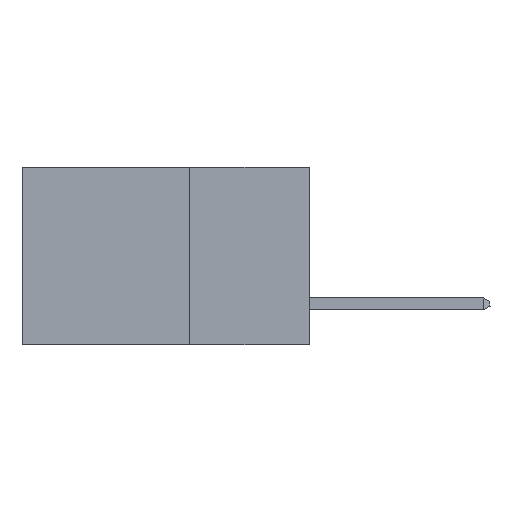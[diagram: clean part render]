
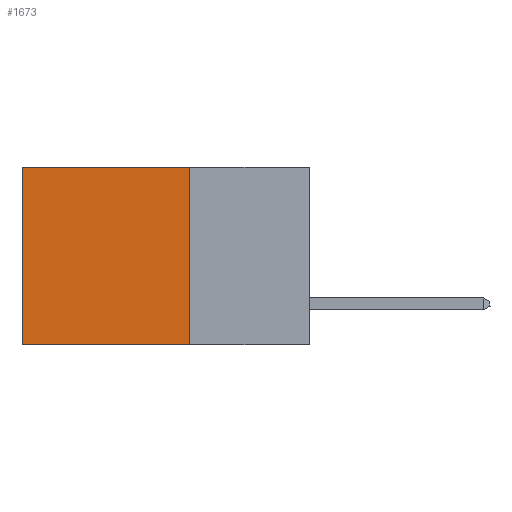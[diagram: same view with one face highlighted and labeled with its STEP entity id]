
A CAD part, left-side view. The second image highlights one B-rep face of the part: STEP entity #1673.
In plain terms, the highlighted planar face has unit normal (-1, 0, 0).
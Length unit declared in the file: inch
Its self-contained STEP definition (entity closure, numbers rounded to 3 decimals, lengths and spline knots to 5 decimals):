
#782 = VERTEX_POINT ( 'NONE', #23137 ) ;
#1673 = ADVANCED_FACE ( 'NONE', ( #12764 ), #16766, .F. ) ;
#4200 = CARTESIAN_POINT ( 'NONE',  ( 0.2875, 0.25, 0. ) ) ;
#4323 = CARTESIAN_POINT ( 'NONE',  ( 0.2875, 0.25, 0. ) ) ;
#4584 = DIRECTION ( 'NONE',  ( 0., 0., -1. ) ) ;
#5018 = EDGE_CURVE ( 'NONE', #782, #20310, #20867, .T. ) ;
#6437 = ORIENTED_EDGE ( 'NONE', *, *, #37140, .T. ) ;
#7591 = ORIENTED_EDGE ( 'NONE', *, *, #28733, .T. ) ;
#7661 = EDGE_LOOP ( 'NONE', ( #7591, #25808, #20550, #6437 ) ) ;
#8180 = EDGE_CURVE ( 'NONE', #14818, #782, #23444, .T. ) ;
#9784 = LINE ( 'NONE', #19017, #10733 ) ;
#10733 = VECTOR ( 'NONE', #37414, 39.37008 ) ;
#12179 = VERTEX_POINT ( 'NONE', #25478 ) ;
#12764 = FACE_OUTER_BOUND ( 'NONE', #7661, .T. ) ;
#14818 = VERTEX_POINT ( 'NONE', #37811 ) ;
#15288 = AXIS2_PLACEMENT_3D ( 'NONE', #22866, #16907, #26030 ) ;
#16766 = PLANE ( 'NONE',  #15288 ) ;
#16907 = DIRECTION ( 'NONE',  ( 1., 0., 0. ) ) ;
#19017 = CARTESIAN_POINT ( 'NONE',  ( 0.2875, 0.6, 0. ) ) ;
#20310 = VERTEX_POINT ( 'NONE', #24332 ) ;
#20550 = ORIENTED_EDGE ( 'NONE', *, *, #8180, .F. ) ;
#20867 = LINE ( 'NONE', #32390, #38370 ) ;
#22866 = CARTESIAN_POINT ( 'NONE',  ( 0.2875, 0.25, 0. ) ) ;
#23137 = CARTESIAN_POINT ( 'NONE',  ( 0.2875, 0.25, -0.37 ) ) ;
#23444 = LINE ( 'NONE', #4323, #24799 ) ;
#24332 = CARTESIAN_POINT ( 'NONE',  ( 0.2875, 0.6, -0.37 ) ) ;
#24799 = VECTOR ( 'NONE', #4584, 39.37008 ) ;
#25078 = DIRECTION ( 'NONE',  ( 0., 1., 0. ) ) ;
#25478 = CARTESIAN_POINT ( 'NONE',  ( 0.2875, 0.6, 0. ) ) ;
#25808 = ORIENTED_EDGE ( 'NONE', *, *, #5018, .F. ) ;
#26030 = DIRECTION ( 'NONE',  ( 0., 0., -1. ) ) ;
#28733 = EDGE_CURVE ( 'NONE', #12179, #20310, #9784, .T. ) ;
#29098 = DIRECTION ( 'NONE',  ( 0., 1., 0. ) ) ;
#30049 = LINE ( 'NONE', #4200, #31039 ) ;
#31039 = VECTOR ( 'NONE', #25078, 39.37008 ) ;
#32390 = CARTESIAN_POINT ( 'NONE',  ( 0.2875, 0.25, -0.37 ) ) ;
#37140 = EDGE_CURVE ( 'NONE', #14818, #12179, #30049, .T. ) ;
#37414 = DIRECTION ( 'NONE',  ( 0., 0., -1. ) ) ;
#37811 = CARTESIAN_POINT ( 'NONE',  ( 0.2875, 0.25, 0. ) ) ;
#38370 = VECTOR ( 'NONE', #29098, 39.37008 ) ;
